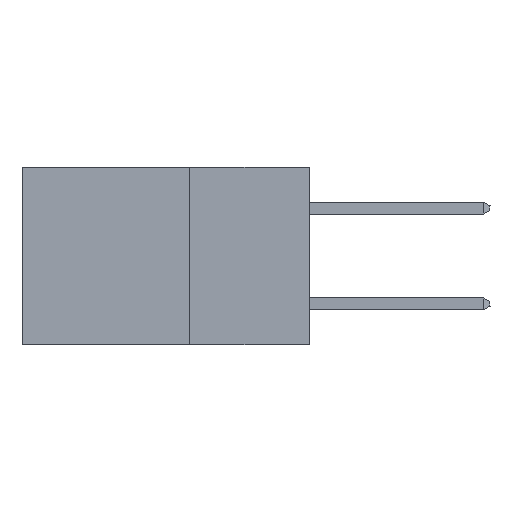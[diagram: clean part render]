
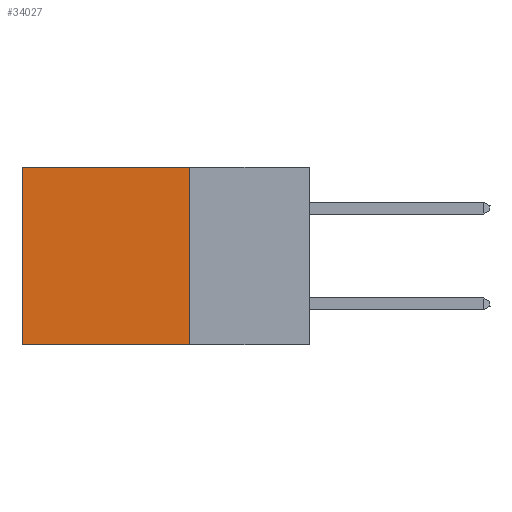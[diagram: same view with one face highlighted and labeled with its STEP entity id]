
A CAD part, left-side view. The second image highlights one B-rep face of the part: STEP entity #34027.
In plain terms, the highlighted planar face has unit normal (-1, 0, 0).
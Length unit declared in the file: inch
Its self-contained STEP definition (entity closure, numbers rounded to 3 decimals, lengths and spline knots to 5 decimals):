
#565 = PLANE ( 'NONE',  #39966 ) ;
#2089 = CARTESIAN_POINT ( 'NONE',  ( 0.2875, 0.25, -0.37 ) ) ;
#3099 = CARTESIAN_POINT ( 'NONE',  ( 0.2875, 0.6, 0. ) ) ;
#3933 = CARTESIAN_POINT ( 'NONE',  ( 0.2875, 0.25, 0. ) ) ;
#4308 = DIRECTION ( 'NONE',  ( 0., 1., 0. ) ) ;
#6204 = LINE ( 'NONE', #3933, #43446 ) ;
#7898 = VERTEX_POINT ( 'NONE', #13109 ) ;
#8346 = VECTOR ( 'NONE', #35220, 39.37008 ) ;
#10702 = EDGE_CURVE ( 'NONE', #38550, #7898, #35464, .T. ) ;
#11401 = CARTESIAN_POINT ( 'NONE',  ( 0.2875, 0.6, 0. ) ) ;
#11668 = VECTOR ( 'NONE', #4308, 39.37008 ) ;
#12020 = VECTOR ( 'NONE', #26210, 39.37008 ) ;
#13109 = CARTESIAN_POINT ( 'NONE',  ( 0.2875, 0.6, -0.37 ) ) ;
#15314 = VERTEX_POINT ( 'NONE', #18529 ) ;
#18529 = CARTESIAN_POINT ( 'NONE',  ( 0.2875, 0.25, 0. ) ) ;
#21419 = CARTESIAN_POINT ( 'NONE',  ( 0.2875, 0.25, 0. ) ) ;
#23212 = EDGE_LOOP ( 'NONE', ( #27761, #43498, #36991, #42739 ) ) ;
#24380 = DIRECTION ( 'NONE',  ( 1., 0., 0. ) ) ;
#25515 = LINE ( 'NONE', #21419, #11668 ) ;
#26210 = DIRECTION ( 'NONE',  ( 0., 1., 0. ) ) ;
#27761 = ORIENTED_EDGE ( 'NONE', *, *, #42194, .T. ) ;
#27762 = FACE_OUTER_BOUND ( 'NONE', #23212, .T. ) ;
#31027 = DIRECTION ( 'NONE',  ( 0., 0., -1. ) ) ;
#31358 = CARTESIAN_POINT ( 'NONE',  ( 0.2875, 0.25, 0. ) ) ;
#32304 = LINE ( 'NONE', #11401, #8346 ) ;
#34027 = ADVANCED_FACE ( 'NONE', ( #27762 ), #565, .F. ) ;
#35220 = DIRECTION ( 'NONE',  ( 0., 0., -1. ) ) ;
#35464 = LINE ( 'NONE', #2089, #12020 ) ;
#36424 = CARTESIAN_POINT ( 'NONE',  ( 0.2875, 0.25, -0.37 ) ) ;
#36991 = ORIENTED_EDGE ( 'NONE', *, *, #37086, .F. ) ;
#37086 = EDGE_CURVE ( 'NONE', #15314, #38550, #6204, .T. ) ;
#37906 = DIRECTION ( 'NONE',  ( 0., 0., -1. ) ) ;
#38550 = VERTEX_POINT ( 'NONE', #36424 ) ;
#39966 = AXIS2_PLACEMENT_3D ( 'NONE', #31358, #24380, #37906 ) ;
#40154 = EDGE_CURVE ( 'NONE', #15314, #41675, #25515, .T. ) ;
#41675 = VERTEX_POINT ( 'NONE', #3099 ) ;
#42194 = EDGE_CURVE ( 'NONE', #41675, #7898, #32304, .T. ) ;
#42739 = ORIENTED_EDGE ( 'NONE', *, *, #40154, .T. ) ;
#43446 = VECTOR ( 'NONE', #31027, 39.37008 ) ;
#43498 = ORIENTED_EDGE ( 'NONE', *, *, #10702, .F. ) ;
